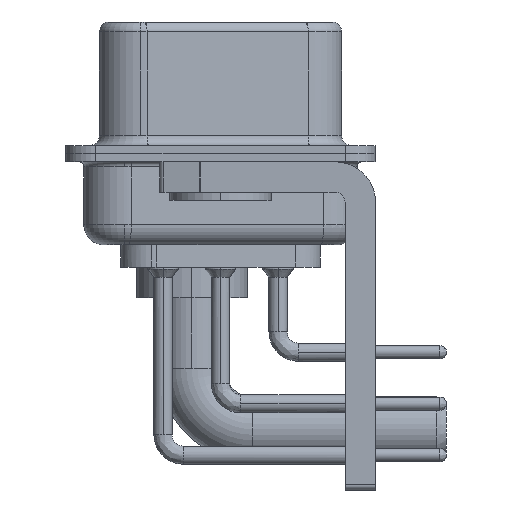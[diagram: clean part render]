
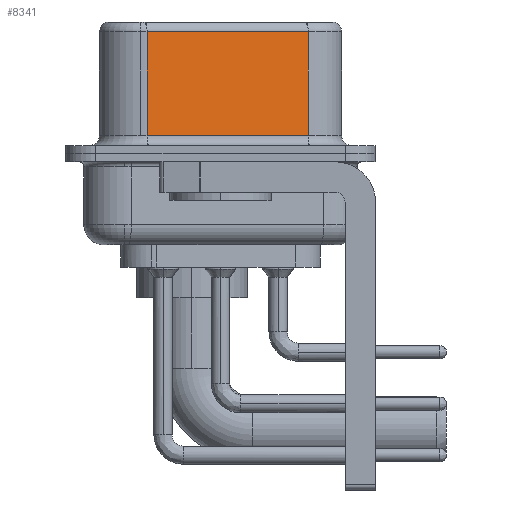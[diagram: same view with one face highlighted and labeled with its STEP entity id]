
A CAD part, left-side view. The second image highlights one B-rep face of the part: STEP entity #8341.
In plain terms, the highlighted planar face has unit normal (-0.985, -0.174, 0).
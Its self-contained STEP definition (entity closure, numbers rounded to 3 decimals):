
#2430 = CARTESIAN_POINT ( 'NONE',  ( 5.132, -4.322, 6.52 ) ) ;
#2502 = AXIS2_PLACEMENT_3D ( 'NONE', #22674, #36507, #16881 ) ;
#2824 = PLANE ( 'NONE',  #2502 ) ;
#3202 = CARTESIAN_POINT ( 'NONE',  ( 3.73, 3.628, 0.9 ) ) ;
#5451 = FACE_OUTER_BOUND ( 'NONE', #28611, .T. ) ;
#8341 = ADVANCED_FACE ( 'NONE', ( #5451 ), #2824, .F. ) ;
#8638 = EDGE_CURVE ( 'NONE', #25908, #15183, #10659, .T. ) ;
#9641 = ORIENTED_EDGE ( 'NONE', *, *, #8638, .T. ) ;
#9930 = LINE ( 'NONE', #35924, #22342 ) ;
#10421 = VERTEX_POINT ( 'NONE', #13241 ) ;
#10659 = LINE ( 'NONE', #29747, #12710 ) ;
#11308 = EDGE_CURVE ( 'NONE', #15183, #21692, #9930, .T. ) ;
#11761 = CARTESIAN_POINT ( 'NONE',  ( 5.132, -4.322, 6.02 ) ) ;
#12710 = VECTOR ( 'NONE', #18728, 1000. ) ;
#12928 = DIRECTION ( 'NONE',  ( 0., 0., -1. ) ) ;
#13241 = CARTESIAN_POINT ( 'NONE',  ( 5.132, -4.322, 0.9 ) ) ;
#13383 = VECTOR ( 'NONE', #13753, 1000. ) ;
#13753 = DIRECTION ( 'NONE',  ( 0.174, -0.985, 0. ) ) ;
#15183 = VERTEX_POINT ( 'NONE', #34274 ) ;
#16881 = DIRECTION ( 'NONE',  ( -0.174, 0.985, 0. ) ) ;
#18728 = DIRECTION ( 'NONE',  ( -0.174, 0.985, 0. ) ) ;
#21692 = VERTEX_POINT ( 'NONE', #3202 ) ;
#22342 = VECTOR ( 'NONE', #12928, 1000. ) ;
#22674 = CARTESIAN_POINT ( 'NONE',  ( 5.132, -4.322, 6.52 ) ) ;
#23682 = ORIENTED_EDGE ( 'NONE', *, *, #29872, .F. ) ;
#25348 = CARTESIAN_POINT ( 'NONE',  ( 5.132, -4.322, 0.9 ) ) ;
#25908 = VERTEX_POINT ( 'NONE', #11761 ) ;
#28322 = LINE ( 'NONE', #25348, #13383 ) ;
#28611 = EDGE_LOOP ( 'NONE', ( #23682, #9641, #34904, #34482 ) ) ;
#28646 = VECTOR ( 'NONE', #36702, 1000. ) ;
#29747 = CARTESIAN_POINT ( 'NONE',  ( 5.132, -4.322, 6.02 ) ) ;
#29872 = EDGE_CURVE ( 'NONE', #25908, #10421, #30898, .T. ) ;
#30898 = LINE ( 'NONE', #2430, #28646 ) ;
#34274 = CARTESIAN_POINT ( 'NONE',  ( 3.73, 3.628, 6.02 ) ) ;
#34482 = ORIENTED_EDGE ( 'NONE', *, *, #35385, .T. ) ;
#34904 = ORIENTED_EDGE ( 'NONE', *, *, #11308, .T. ) ;
#35385 = EDGE_CURVE ( 'NONE', #21692, #10421, #28322, .T. ) ;
#35924 = CARTESIAN_POINT ( 'NONE',  ( 3.73, 3.628, 6.52 ) ) ;
#36507 = DIRECTION ( 'NONE',  ( 0.985, 0.174, 0. ) ) ;
#36702 = DIRECTION ( 'NONE',  ( 0., 0., -1. ) ) ;
